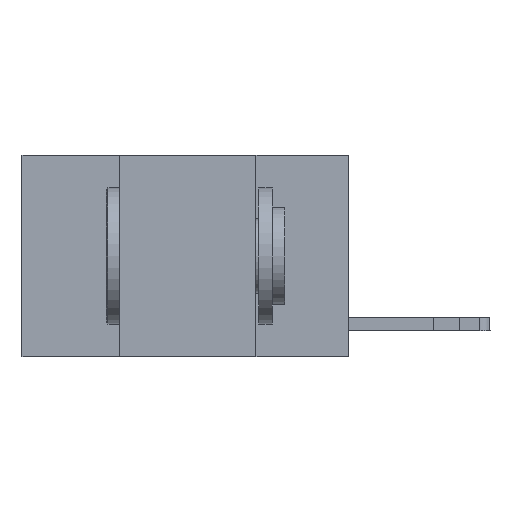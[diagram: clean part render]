
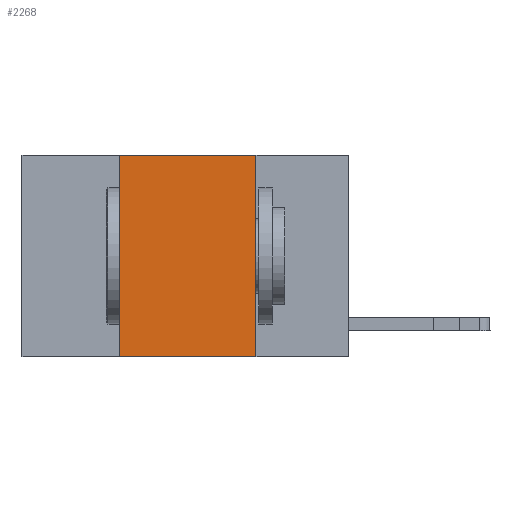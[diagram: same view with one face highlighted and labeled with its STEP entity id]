
A CAD part, left-side view. The second image highlights one B-rep face of the part: STEP entity #2268.
In plain terms, the highlighted planar face has unit normal (-1, 0, 0).
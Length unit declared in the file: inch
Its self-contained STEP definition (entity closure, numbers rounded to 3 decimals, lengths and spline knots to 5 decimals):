
#512 = EDGE_CURVE ( 'NONE', #19784, #4753, #8173, .T. ) ;
#774 = VERTEX_POINT ( 'NONE', #14015 ) ;
#2268 = ADVANCED_FACE ( 'NONE', ( #16545 ), #9938, .F. ) ;
#2333 = CARTESIAN_POINT ( 'NONE',  ( 0., 0.6, -0.37 ) ) ;
#3087 = ORIENTED_EDGE ( 'NONE', *, *, #19911, .T. ) ;
#3115 = EDGE_LOOP ( 'NONE', ( #22401, #9537, #16061, #3087 ) ) ;
#3313 = DIRECTION ( 'NONE',  ( 0., 0., 1. ) ) ;
#4753 = VERTEX_POINT ( 'NONE', #6162 ) ;
#5967 = AXIS2_PLACEMENT_3D ( 'NONE', #14819, #16658, #20230 ) ;
#6162 = CARTESIAN_POINT ( 'NONE',  ( 0., 0.17, 0. ) ) ;
#6722 = VECTOR ( 'NONE', #22064, 39.37008 ) ;
#7087 = EDGE_CURVE ( 'NONE', #10375, #19784, #12193, .T. ) ;
#8173 = LINE ( 'NONE', #15224, #20200 ) ;
#8467 = CARTESIAN_POINT ( 'NONE',  ( 0., 0.17, 0. ) ) ;
#9134 = CARTESIAN_POINT ( 'NONE',  ( 0., 0.42, -0.37 ) ) ;
#9243 = LINE ( 'NONE', #2333, #6722 ) ;
#9537 = ORIENTED_EDGE ( 'NONE', *, *, #512, .F. ) ;
#9938 = PLANE ( 'NONE',  #5967 ) ;
#10205 = EDGE_CURVE ( 'NONE', #4753, #774, #19220, .T. ) ;
#10375 = VERTEX_POINT ( 'NONE', #9134 ) ;
#11684 = VECTOR ( 'NONE', #3313, 39.37008 ) ;
#12193 = LINE ( 'NONE', #15883, #11684 ) ;
#14015 = CARTESIAN_POINT ( 'NONE',  ( 0., 0.17, -0.37 ) ) ;
#14819 = CARTESIAN_POINT ( 'NONE',  ( 0., 0.6, 0. ) ) ;
#15224 = CARTESIAN_POINT ( 'NONE',  ( 0., 0.6, 0. ) ) ;
#15519 = DIRECTION ( 'NONE',  ( 0., 0., -1. ) ) ;
#15883 = CARTESIAN_POINT ( 'NONE',  ( 0., 0.42, 0. ) ) ;
#16061 = ORIENTED_EDGE ( 'NONE', *, *, #7087, .F. ) ;
#16166 = CARTESIAN_POINT ( 'NONE',  ( 0., 0.42, 0. ) ) ;
#16545 = FACE_OUTER_BOUND ( 'NONE', #3115, .T. ) ;
#16658 = DIRECTION ( 'NONE',  ( 1., 0., 0. ) ) ;
#19220 = LINE ( 'NONE', #8467, #21247 ) ;
#19784 = VERTEX_POINT ( 'NONE', #16166 ) ;
#19911 = EDGE_CURVE ( 'NONE', #10375, #774, #9243, .T. ) ;
#20200 = VECTOR ( 'NONE', #22262, 39.37008 ) ;
#20230 = DIRECTION ( 'NONE',  ( 0., 0., -1. ) ) ;
#21247 = VECTOR ( 'NONE', #15519, 39.37008 ) ;
#22064 = DIRECTION ( 'NONE',  ( 0., -1., 0. ) ) ;
#22262 = DIRECTION ( 'NONE',  ( 0., -1., 0. ) ) ;
#22401 = ORIENTED_EDGE ( 'NONE', *, *, #10205, .F. ) ;
